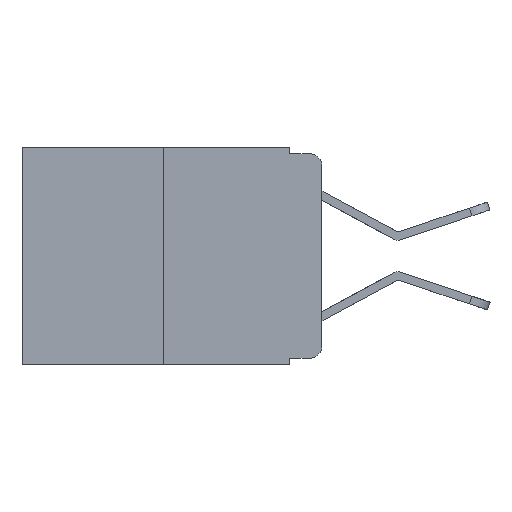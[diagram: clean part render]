
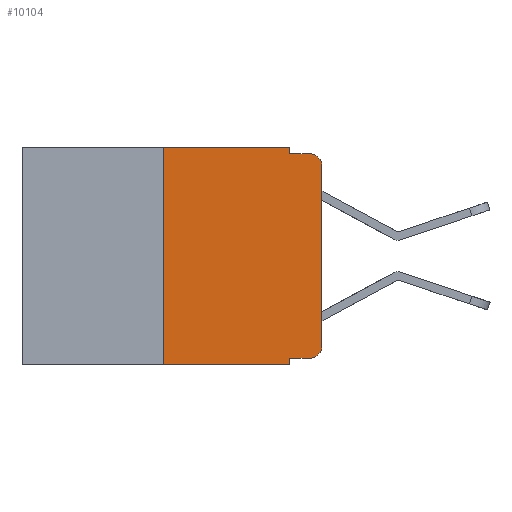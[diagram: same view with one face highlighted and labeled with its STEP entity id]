
A CAD part, left-side view. The second image highlights one B-rep face of the part: STEP entity #10104.
In plain terms, the highlighted planar face has unit normal (-1, 0, 0).
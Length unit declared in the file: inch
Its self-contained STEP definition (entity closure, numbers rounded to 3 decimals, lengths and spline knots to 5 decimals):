
#84 = LINE ( 'NONE', #5519, #13278 ) ;
#494 = ORIENTED_EDGE ( 'NONE', *, *, #1369, .F. ) ;
#516 = CARTESIAN_POINT ( 'NONE',  ( 0., 0.051, -0.343 ) ) ;
#553 = VERTEX_POINT ( 'NONE', #2209 ) ;
#612 = ORIENTED_EDGE ( 'NONE', *, *, #9602, .T. ) ;
#645 = LINE ( 'NONE', #15626, #7156 ) ;
#871 = AXIS2_PLACEMENT_3D ( 'NONE', #9919, #10754, #14985 ) ;
#879 = VECTOR ( 'NONE', #10549, 39.37008 ) ;
#1009 = CARTESIAN_POINT ( 'NONE',  ( 0., 0.25, -0.343 ) ) ;
#1044 = CARTESIAN_POINT ( 'NONE',  ( 0., 0.051, 0. ) ) ;
#1127 = CARTESIAN_POINT ( 'NONE',  ( 0., 0.02, -0.03 ) ) ;
#1131 = CARTESIAN_POINT ( 'NONE',  ( 0., 0.051, 0. ) ) ;
#1206 = CARTESIAN_POINT ( 'NONE',  ( 0., 0.02, -0.01 ) ) ;
#1369 = EDGE_CURVE ( 'NONE', #11622, #3353, #645, .T. ) ;
#1673 = DIRECTION ( 'NONE',  ( 0., 0., -1. ) ) ;
#1931 = VERTEX_POINT ( 'NONE', #7741 ) ;
#2058 = ORIENTED_EDGE ( 'NONE', *, *, #5931, .F. ) ;
#2196 = CARTESIAN_POINT ( 'NONE',  ( 0., 0.473, 0. ) ) ;
#2209 = CARTESIAN_POINT ( 'NONE',  ( 0., 0.051, -0.333 ) ) ;
#2385 = LINE ( 'NONE', #1131, #879 ) ;
#2641 = DIRECTION ( 'NONE',  ( 0., 0., -1. ) ) ;
#2710 = ORIENTED_EDGE ( 'NONE', *, *, #12728, .T. ) ;
#2840 = CIRCLE ( 'NONE', #15939, 0.02 ) ;
#3353 = VERTEX_POINT ( 'NONE', #12717 ) ;
#3533 = LINE ( 'NONE', #14415, #5701 ) ;
#4011 = ORIENTED_EDGE ( 'NONE', *, *, #5111, .T. ) ;
#4244 = ORIENTED_EDGE ( 'NONE', *, *, #14278, .F. ) ;
#4369 = CARTESIAN_POINT ( 'NONE',  ( 0., 0., -0.313 ) ) ;
#4412 = EDGE_CURVE ( 'NONE', #553, #1931, #15448, .T. ) ;
#4506 = PLANE ( 'NONE',  #871 ) ;
#4603 = ORIENTED_EDGE ( 'NONE', *, *, #13650, .T. ) ;
#4703 = DIRECTION ( 'NONE',  ( 0., 0., 1. ) ) ;
#5111 = EDGE_CURVE ( 'NONE', #11622, #7755, #9917, .T. ) ;
#5519 = CARTESIAN_POINT ( 'NONE',  ( 0., 0.051, -0.01 ) ) ;
#5701 = VECTOR ( 'NONE', #4703, 39.37008 ) ;
#5821 = VECTOR ( 'NONE', #8497, 39.37008 ) ;
#5931 = EDGE_CURVE ( 'NONE', #6136, #9775, #84, .T. ) ;
#5946 = DIRECTION ( 'NONE',  ( -1., 0., 0. ) ) ;
#5963 = VECTOR ( 'NONE', #12893, 39.37008 ) ;
#6136 = VERTEX_POINT ( 'NONE', #11479 ) ;
#6408 = FACE_OUTER_BOUND ( 'NONE', #11984, .T. ) ;
#6808 = DIRECTION ( 'NONE',  ( -1., 0., 0. ) ) ;
#7156 = VECTOR ( 'NONE', #10248, 39.37008 ) ;
#7741 = CARTESIAN_POINT ( 'NONE',  ( 0., 0.02, -0.333 ) ) ;
#7755 = VERTEX_POINT ( 'NONE', #516 ) ;
#7793 = CARTESIAN_POINT ( 'NONE',  ( 0., 0.051, 0. ) ) ;
#8497 = DIRECTION ( 'NONE',  ( 0., -1., 0. ) ) ;
#9340 = ORIENTED_EDGE ( 'NONE', *, *, #4412, .T. ) ;
#9602 = EDGE_CURVE ( 'NONE', #12412, #12943, #3533, .T. ) ;
#9775 = VERTEX_POINT ( 'NONE', #1206 ) ;
#9917 = LINE ( 'NONE', #16812, #5821 ) ;
#9919 = CARTESIAN_POINT ( 'NONE',  ( 0., 0.473, 0. ) ) ;
#9969 = ORIENTED_EDGE ( 'NONE', *, *, #14336, .F. ) ;
#10104 = ADVANCED_FACE ( 'NONE', ( #6408 ), #4506, .F. ) ;
#10248 = DIRECTION ( 'NONE',  ( 0., 0., 1. ) ) ;
#10312 = VECTOR ( 'NONE', #12939, 39.37008 ) ;
#10366 = LINE ( 'NONE', #7793, #5963 ) ;
#10549 = DIRECTION ( 'NONE',  ( 0., 0., -1. ) ) ;
#10754 = DIRECTION ( 'NONE',  ( 1., 0., 0. ) ) ;
#10982 = VERTEX_POINT ( 'NONE', #1044 ) ;
#11369 = VECTOR ( 'NONE', #13156, 39.37008 ) ;
#11479 = CARTESIAN_POINT ( 'NONE',  ( 0., 0.051, -0.01 ) ) ;
#11537 = CARTESIAN_POINT ( 'NONE',  ( 0., 0., -0.03 ) ) ;
#11622 = VERTEX_POINT ( 'NONE', #1009 ) ;
#11984 = EDGE_LOOP ( 'NONE', ( #612, #2710, #2058, #9969, #4244, #494, #4011, #15835, #9340, #4603 ) ) ;
#12412 = VERTEX_POINT ( 'NONE', #4369 ) ;
#12473 = AXIS2_PLACEMENT_3D ( 'NONE', #1127, #6808, #2641 ) ;
#12717 = CARTESIAN_POINT ( 'NONE',  ( 0., 0.25, 0. ) ) ;
#12728 = EDGE_CURVE ( 'NONE', #12943, #9775, #13910, .T. ) ;
#12893 = DIRECTION ( 'NONE',  ( 0., 0., -1. ) ) ;
#12939 = DIRECTION ( 'NONE',  ( 0., -1., 0. ) ) ;
#12943 = VERTEX_POINT ( 'NONE', #11537 ) ;
#13156 = DIRECTION ( 'NONE',  ( 0., -1., 0. ) ) ;
#13278 = VECTOR ( 'NONE', #14002, 39.37008 ) ;
#13650 = EDGE_CURVE ( 'NONE', #1931, #12412, #2840, .T. ) ;
#13910 = CIRCLE ( 'NONE', #12473, 0.02 ) ;
#13993 = CARTESIAN_POINT ( 'NONE',  ( 0., 0.02, -0.313 ) ) ;
#14002 = DIRECTION ( 'NONE',  ( 0., -1., 0. ) ) ;
#14278 = EDGE_CURVE ( 'NONE', #3353, #10982, #14570, .T. ) ;
#14336 = EDGE_CURVE ( 'NONE', #10982, #6136, #10366, .T. ) ;
#14415 = CARTESIAN_POINT ( 'NONE',  ( 0., 0., 0. ) ) ;
#14570 = LINE ( 'NONE', #2196, #11369 ) ;
#14985 = DIRECTION ( 'NONE',  ( 0., 0., -1. ) ) ;
#15448 = LINE ( 'NONE', #15535, #10312 ) ;
#15535 = CARTESIAN_POINT ( 'NONE',  ( 0., 0.051, -0.333 ) ) ;
#15626 = CARTESIAN_POINT ( 'NONE',  ( 0., 0.25, 0. ) ) ;
#15835 = ORIENTED_EDGE ( 'NONE', *, *, #16777, .F. ) ;
#15939 = AXIS2_PLACEMENT_3D ( 'NONE', #13993, #5946, #1673 ) ;
#16777 = EDGE_CURVE ( 'NONE', #553, #7755, #2385, .T. ) ;
#16812 = CARTESIAN_POINT ( 'NONE',  ( 0., 0.473, -0.343 ) ) ;
